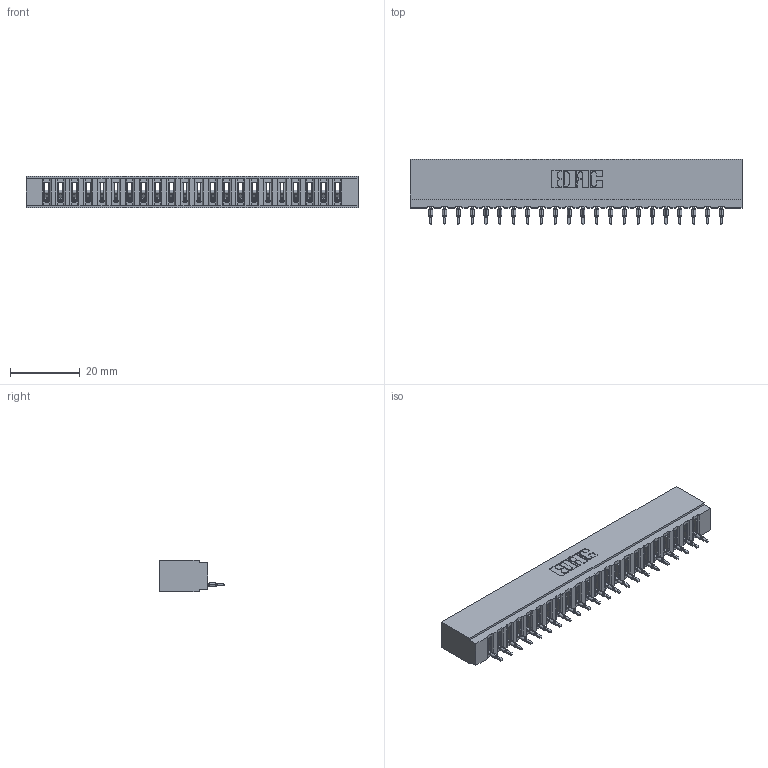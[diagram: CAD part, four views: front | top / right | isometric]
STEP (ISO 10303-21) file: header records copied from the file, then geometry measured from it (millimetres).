
FILE_DESCRIPTION (( 'STEP AP203' ), '1' );
FILE_NAME ('717-022-560-106.STEP', '2020-03-13T19:26:15', ( '' ), ( '' ), 'SwSTEP 2.0', 'SolidWorks 2016', '' );
FILE_SCHEMA (( 'CONFIG_CONTROL_DESIGN' ));
Length unit declared in the file: inch
Products named in the file (3): 717-022-560-106; 745-292-001_560; 717 Part_Insulator Option - 06
Assembly tree (23 placements, depth 2):
  717-022-560-106
    717 Part_Insulator Option - 06
    745-292-001_560  x22
Bounding box: 95.05 x 18.78 x 8.89 mm (x, y, z)
Volume: 8184.2 mm3; surface area: 11635.5 mm2
Topology: 23 solids, 23 shells, 2778 faces, 7731 edges, 4918 vertices
Faces by surface type: plane 1660, cylinder 546, bspline 440, torus 132
Entity records: 40050 total; most frequent: CARTESIAN_POINT 7561, ORIENTED_EDGE 6978, DIRECTION 6071, EDGE_CURVE 3489, VECTOR 3167, LINE 3167, VERTEX_POINT 2230, AXIS2_PLACEMENT_3D 1452
